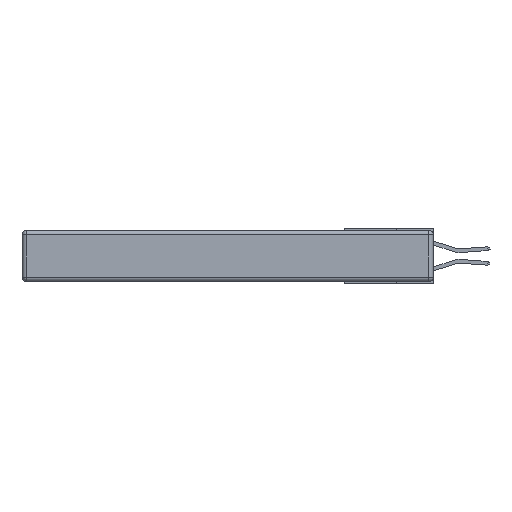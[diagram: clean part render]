
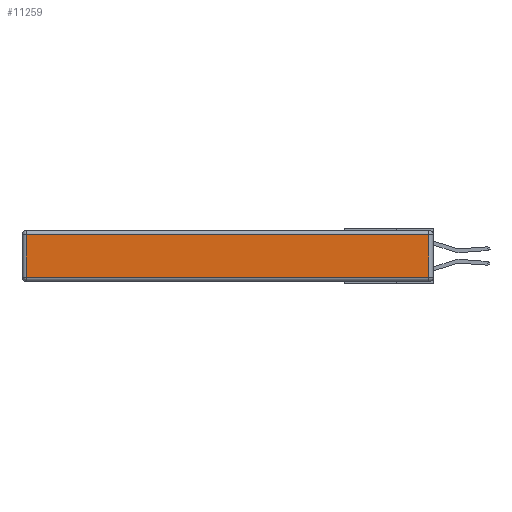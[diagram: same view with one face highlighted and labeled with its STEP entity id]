
A CAD part, left-side view. The second image highlights one B-rep face of the part: STEP entity #11259.
In plain terms, the highlighted planar face has unit normal (-1, 0, 0).
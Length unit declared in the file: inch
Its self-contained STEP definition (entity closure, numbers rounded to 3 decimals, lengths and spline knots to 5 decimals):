
#440 = CARTESIAN_POINT ( 'NONE',  ( 0., 2.72, -0.343 ) ) ;
#707 = CARTESIAN_POINT ( 'NONE',  ( 0., 0.03, -0.03 ) ) ;
#1201 = CARTESIAN_POINT ( 'NONE',  ( 0., 2.72, -0.313 ) ) ;
#1207 = ORIENTED_EDGE ( 'NONE', *, *, #7637, .T. ) ;
#1971 = CARTESIAN_POINT ( 'NONE',  ( 0., 0., -0.343 ) ) ;
#2246 = AXIS2_PLACEMENT_3D ( 'NONE', #1971, #3813, #8807 ) ;
#2844 = LINE ( 'NONE', #7540, #12454 ) ;
#2918 = CARTESIAN_POINT ( 'NONE',  ( 0., 2.72, -0.03 ) ) ;
#3650 = ORIENTED_EDGE ( 'NONE', *, *, #7433, .T. ) ;
#3813 = DIRECTION ( 'NONE',  ( -1., 0., 0. ) ) ;
#3838 = CARTESIAN_POINT ( 'NONE',  ( 0., 0.03, -0.343 ) ) ;
#3918 = DIRECTION ( 'NONE',  ( 0., 1., 0. ) ) ;
#4737 = PLANE ( 'NONE',  #2246 ) ;
#4977 = LINE ( 'NONE', #3838, #9133 ) ;
#5172 = LINE ( 'NONE', #440, #7340 ) ;
#5557 = EDGE_LOOP ( 'NONE', ( #1207, #6113, #9790, #3650 ) ) ;
#5940 = VECTOR ( 'NONE', #3918, 39.37008 ) ;
#6113 = ORIENTED_EDGE ( 'NONE', *, *, #8795, .T. ) ;
#6144 = FACE_OUTER_BOUND ( 'NONE', #5557, .T. ) ;
#6410 = VERTEX_POINT ( 'NONE', #2918 ) ;
#6418 = EDGE_CURVE ( 'NONE', #9004, #6410, #8701, .T. ) ;
#7123 = VERTEX_POINT ( 'NONE', #12384 ) ;
#7340 = VECTOR ( 'NONE', #11061, 39.37008 ) ;
#7433 = EDGE_CURVE ( 'NONE', #6410, #7507, #5172, .T. ) ;
#7507 = VERTEX_POINT ( 'NONE', #1201 ) ;
#7540 = CARTESIAN_POINT ( 'NONE',  ( 0., 0., -0.313 ) ) ;
#7637 = EDGE_CURVE ( 'NONE', #7507, #7123, #2844, .T. ) ;
#8518 = DIRECTION ( 'NONE',  ( 0., -1., 0. ) ) ;
#8701 = LINE ( 'NONE', #8869, #5940 ) ;
#8785 = DIRECTION ( 'NONE',  ( 0., 0., 1. ) ) ;
#8795 = EDGE_CURVE ( 'NONE', #7123, #9004, #4977, .T. ) ;
#8807 = DIRECTION ( 'NONE',  ( 0., 0., 1. ) ) ;
#8869 = CARTESIAN_POINT ( 'NONE',  ( 0., 2.75, -0.03 ) ) ;
#9004 = VERTEX_POINT ( 'NONE', #707 ) ;
#9133 = VECTOR ( 'NONE', #8785, 39.37008 ) ;
#9790 = ORIENTED_EDGE ( 'NONE', *, *, #6418, .T. ) ;
#11061 = DIRECTION ( 'NONE',  ( 0., 0., -1. ) ) ;
#11259 = ADVANCED_FACE ( 'NONE', ( #6144 ), #4737, .T. ) ;
#12384 = CARTESIAN_POINT ( 'NONE',  ( 0., 0.03, -0.313 ) ) ;
#12454 = VECTOR ( 'NONE', #8518, 39.37008 ) ;
